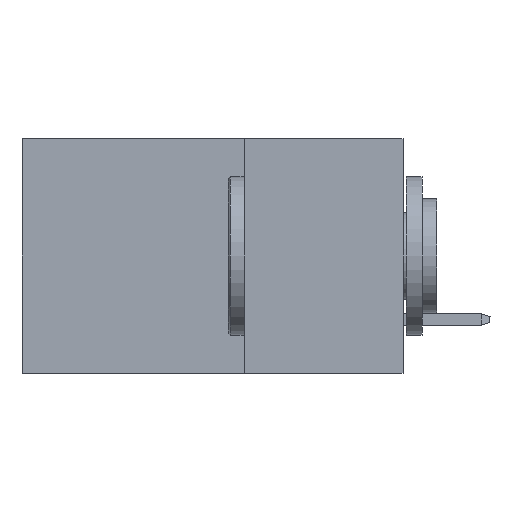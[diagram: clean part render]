
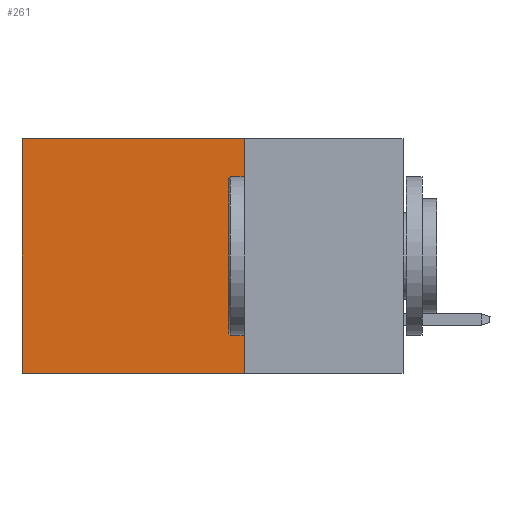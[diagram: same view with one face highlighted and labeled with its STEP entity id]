
A CAD part, left-side view. The second image highlights one B-rep face of the part: STEP entity #261.
In plain terms, the highlighted planar face has unit normal (-1, 0, 0).
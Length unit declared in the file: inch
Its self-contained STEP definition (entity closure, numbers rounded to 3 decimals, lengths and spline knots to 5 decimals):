
#261 = ADVANCED_FACE ( 'NONE', ( #25989 ), #25634, .F. ) ;
#614 = LINE ( 'NONE', #25236, #8257 ) ;
#639 = EDGE_CURVE ( 'NONE', #21329, #26180, #6414, .T. ) ;
#1048 = LINE ( 'NONE', #14933, #20935 ) ;
#1400 = CARTESIAN_POINT ( 'NONE',  ( 0.2875, 0.25, 0. ) ) ;
#1480 = ORIENTED_EDGE ( 'NONE', *, *, #12674, .F. ) ;
#3653 = DIRECTION ( 'NONE',  ( 0., 1., 0. ) ) ;
#3914 = CARTESIAN_POINT ( 'NONE',  ( 0.2875, 0.25, 0. ) ) ;
#5949 = DIRECTION ( 'NONE',  ( 1., 0., 0. ) ) ;
#6414 = LINE ( 'NONE', #28669, #27796 ) ;
#6522 = LINE ( 'NONE', #28950, #31727 ) ;
#8257 = VECTOR ( 'NONE', #11758, 39.37008 ) ;
#10755 = EDGE_CURVE ( 'NONE', #29503, #26180, #1048, .T. ) ;
#11758 = DIRECTION ( 'NONE',  ( 0., 0., -1. ) ) ;
#12674 = EDGE_CURVE ( 'NONE', #14073, #21329, #614, .T. ) ;
#14073 = VERTEX_POINT ( 'NONE', #1400 ) ;
#14933 = CARTESIAN_POINT ( 'NONE',  ( 0.2875, 0.6, 0. ) ) ;
#15049 = CARTESIAN_POINT ( 'NONE',  ( 0.2875, 0.6, 0. ) ) ;
#15717 = EDGE_CURVE ( 'NONE', #14073, #29503, #6522, .T. ) ;
#17064 = DIRECTION ( 'NONE',  ( 0., 0., -1. ) ) ;
#20170 = DIRECTION ( 'NONE',  ( 0., 1., 0. ) ) ;
#20520 = CARTESIAN_POINT ( 'NONE',  ( 0.2875, 0.25, -0.37 ) ) ;
#20935 = VECTOR ( 'NONE', #23294, 39.37008 ) ;
#21329 = VERTEX_POINT ( 'NONE', #20520 ) ;
#21452 = CARTESIAN_POINT ( 'NONE',  ( 0.2875, 0.6, -0.37 ) ) ;
#22454 = ORIENTED_EDGE ( 'NONE', *, *, #15717, .T. ) ;
#22653 = ORIENTED_EDGE ( 'NONE', *, *, #639, .F. ) ;
#23294 = DIRECTION ( 'NONE',  ( 0., 0., -1. ) ) ;
#25236 = CARTESIAN_POINT ( 'NONE',  ( 0.2875, 0.25, 0. ) ) ;
#25634 = PLANE ( 'NONE',  #26692 ) ;
#25989 = FACE_OUTER_BOUND ( 'NONE', #28661, .T. ) ;
#26180 = VERTEX_POINT ( 'NONE', #21452 ) ;
#26692 = AXIS2_PLACEMENT_3D ( 'NONE', #3914, #5949, #17064 ) ;
#27796 = VECTOR ( 'NONE', #3653, 39.37008 ) ;
#28661 = EDGE_LOOP ( 'NONE', ( #35608, #22653, #1480, #22454 ) ) ;
#28669 = CARTESIAN_POINT ( 'NONE',  ( 0.2875, 0.25, -0.37 ) ) ;
#28950 = CARTESIAN_POINT ( 'NONE',  ( 0.2875, 0.25, 0. ) ) ;
#29503 = VERTEX_POINT ( 'NONE', #15049 ) ;
#31727 = VECTOR ( 'NONE', #20170, 39.37008 ) ;
#35608 = ORIENTED_EDGE ( 'NONE', *, *, #10755, .T. ) ;
